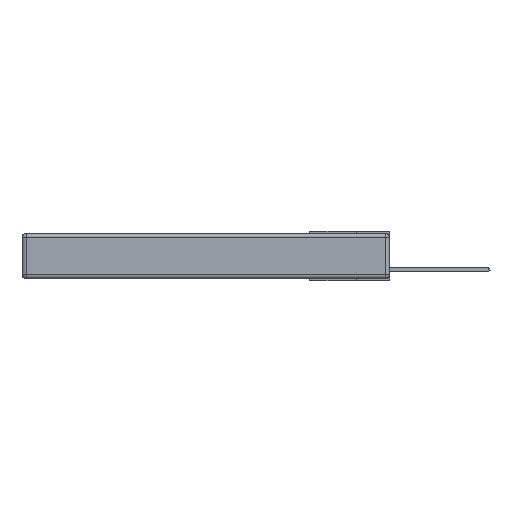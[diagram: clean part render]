
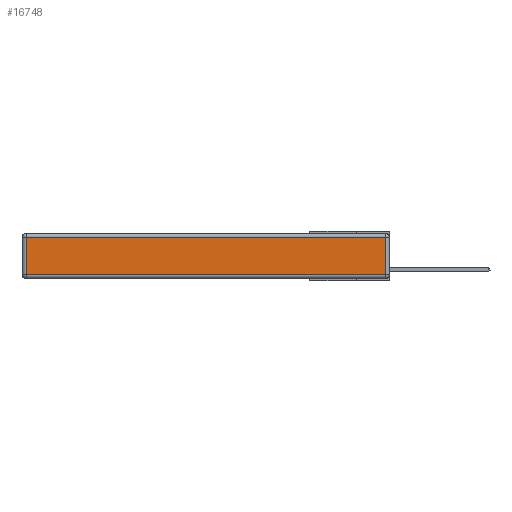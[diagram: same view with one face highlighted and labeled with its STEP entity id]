
A CAD part, left-side view. The second image highlights one B-rep face of the part: STEP entity #16748.
In plain terms, the highlighted planar face has unit normal (-1, 0, 0).
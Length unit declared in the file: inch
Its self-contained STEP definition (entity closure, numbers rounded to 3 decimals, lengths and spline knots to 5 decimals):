
#357 = ORIENTED_EDGE ( 'NONE', *, *, #10017, .T. ) ;
#873 = LINE ( 'NONE', #11571, #21483 ) ;
#1441 = DIRECTION ( 'NONE',  ( 0., 0., -1. ) ) ;
#2003 = LINE ( 'NONE', #11344, #9095 ) ;
#2030 = CARTESIAN_POINT ( 'NONE',  ( 0., 0.03, -0.343 ) ) ;
#2085 = CARTESIAN_POINT ( 'NONE',  ( 0., 0., -0.343 ) ) ;
#2360 = FACE_OUTER_BOUND ( 'NONE', #11118, .T. ) ;
#3085 = ORIENTED_EDGE ( 'NONE', *, *, #8125, .T. ) ;
#3926 = ORIENTED_EDGE ( 'NONE', *, *, #16263, .T. ) ;
#4673 = CARTESIAN_POINT ( 'NONE',  ( 0., 0.03, -0.03 ) ) ;
#5366 = VERTEX_POINT ( 'NONE', #5945 ) ;
#5464 = DIRECTION ( 'NONE',  ( 0., 0., 1. ) ) ;
#5945 = CARTESIAN_POINT ( 'NONE',  ( 0., 2.72, -0.03 ) ) ;
#6119 = DIRECTION ( 'NONE',  ( 0., -1., 0. ) ) ;
#7531 = PLANE ( 'NONE',  #12053 ) ;
#8125 = EDGE_CURVE ( 'NONE', #10891, #16961, #21912, .T. ) ;
#9095 = VECTOR ( 'NONE', #6119, 39.37008 ) ;
#9198 = DIRECTION ( 'NONE',  ( -1., 0., 0. ) ) ;
#9855 = CARTESIAN_POINT ( 'NONE',  ( 0., 2.72, -0.343 ) ) ;
#10017 = EDGE_CURVE ( 'NONE', #5366, #22200, #18141, .T. ) ;
#10734 = VECTOR ( 'NONE', #1441, 39.37008 ) ;
#10866 = CARTESIAN_POINT ( 'NONE',  ( 0., 2.72, -0.313 ) ) ;
#10891 = VERTEX_POINT ( 'NONE', #12095 ) ;
#11118 = EDGE_LOOP ( 'NONE', ( #3926, #3085, #11243, #357 ) ) ;
#11243 = ORIENTED_EDGE ( 'NONE', *, *, #19231, .T. ) ;
#11344 = CARTESIAN_POINT ( 'NONE',  ( 0., 0., -0.313 ) ) ;
#11571 = CARTESIAN_POINT ( 'NONE',  ( 0., 2.75, -0.03 ) ) ;
#12053 = AXIS2_PLACEMENT_3D ( 'NONE', #2085, #9198, #5464 ) ;
#12095 = CARTESIAN_POINT ( 'NONE',  ( 0., 0.03, -0.313 ) ) ;
#14465 = DIRECTION ( 'NONE',  ( 0., 0., 1. ) ) ;
#16263 = EDGE_CURVE ( 'NONE', #22200, #10891, #2003, .T. ) ;
#16748 = ADVANCED_FACE ( 'NONE', ( #2360 ), #7531, .T. ) ;
#16961 = VERTEX_POINT ( 'NONE', #4673 ) ;
#18141 = LINE ( 'NONE', #9855, #10734 ) ;
#19231 = EDGE_CURVE ( 'NONE', #16961, #5366, #873, .T. ) ;
#20402 = DIRECTION ( 'NONE',  ( 0., 1., 0. ) ) ;
#21483 = VECTOR ( 'NONE', #20402, 39.37008 ) ;
#21912 = LINE ( 'NONE', #2030, #22731 ) ;
#22200 = VERTEX_POINT ( 'NONE', #10866 ) ;
#22731 = VECTOR ( 'NONE', #14465, 39.37008 ) ;
